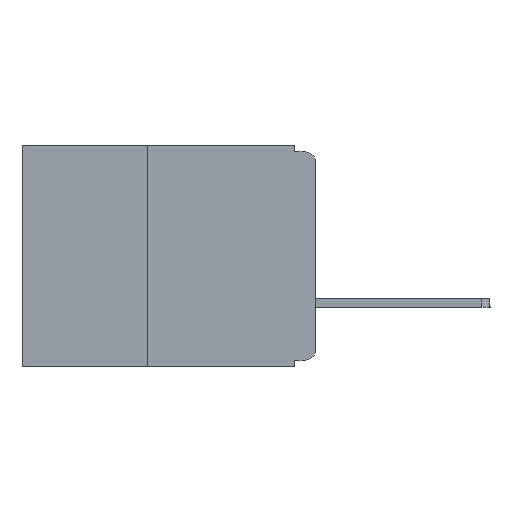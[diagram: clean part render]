
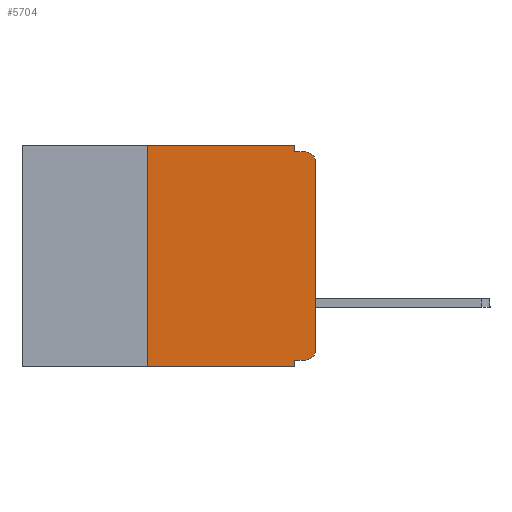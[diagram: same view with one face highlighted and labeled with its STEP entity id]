
A CAD part, left-side view. The second image highlights one B-rep face of the part: STEP entity #5704.
In plain terms, the highlighted planar face has unit normal (-1, 0, 0).
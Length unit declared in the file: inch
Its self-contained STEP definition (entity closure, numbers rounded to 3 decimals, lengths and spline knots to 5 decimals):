
#162 = EDGE_CURVE ( 'NONE', #481, #22862, #1469, .T. ) ;
#481 = VERTEX_POINT ( 'NONE', #14694 ) ;
#590 = VERTEX_POINT ( 'NONE', #20895 ) ;
#1469 = LINE ( 'NONE', #8466, #20929 ) ;
#1602 = EDGE_CURVE ( 'NONE', #24360, #5163, #13462, .T. ) ;
#1803 = ORIENTED_EDGE ( 'NONE', *, *, #17108, .F. ) ;
#2647 = EDGE_CURVE ( 'NONE', #15593, #23224, #3702, .T. ) ;
#2876 = DIRECTION ( 'NONE',  ( 0., 0., -1. ) ) ;
#3011 = DIRECTION ( 'NONE',  ( -1., 0., 0. ) ) ;
#3167 = CARTESIAN_POINT ( 'NONE',  ( 0., 0.015, -0.025 ) ) ;
#3227 = ORIENTED_EDGE ( 'NONE', *, *, #11459, .F. ) ;
#3702 = LINE ( 'NONE', #5252, #23172 ) ;
#3793 = VECTOR ( 'NONE', #11118, 39.37008 ) ;
#4370 = CARTESIAN_POINT ( 'NONE',  ( 0., 0.031, -0.33 ) ) ;
#4485 = DIRECTION ( 'NONE',  ( 1., 0., 0. ) ) ;
#5112 = DIRECTION ( 'NONE',  ( 0., 0., -1. ) ) ;
#5163 = VERTEX_POINT ( 'NONE', #10400 ) ;
#5252 = CARTESIAN_POINT ( 'NONE',  ( 0., 0., -0.32 ) ) ;
#5704 = ADVANCED_FACE ( 'NONE', ( #7215 ), #13904, .F. ) ;
#6299 = LINE ( 'NONE', #12323, #10757 ) ;
#7215 = FACE_OUTER_BOUND ( 'NONE', #22730, .T. ) ;
#7368 = CARTESIAN_POINT ( 'NONE',  ( 0., 0.031, -0.33 ) ) ;
#8285 = CARTESIAN_POINT ( 'NONE',  ( 0., 0.031, -0.01 ) ) ;
#8466 = CARTESIAN_POINT ( 'NONE',  ( 0., 0.031, 0. ) ) ;
#8816 = CARTESIAN_POINT ( 'NONE',  ( 0., 0.015, -0.305 ) ) ;
#9019 = VERTEX_POINT ( 'NONE', #7368 ) ;
#9244 = LINE ( 'NONE', #20651, #13685 ) ;
#9420 = AXIS2_PLACEMENT_3D ( 'NONE', #17643, #4485, #17721 ) ;
#9978 = EDGE_CURVE ( 'NONE', #15593, #12582, #23554, .T. ) ;
#9984 = LINE ( 'NONE', #13080, #19439 ) ;
#10085 = DIRECTION ( 'NONE',  ( 0., 0., -1. ) ) ;
#10152 = AXIS2_PLACEMENT_3D ( 'NONE', #3167, #3011, #2876 ) ;
#10177 = EDGE_CURVE ( 'NONE', #12582, #24360, #9984, .T. ) ;
#10400 = CARTESIAN_POINT ( 'NONE',  ( 0., 0.015, -0.01 ) ) ;
#10725 = DIRECTION ( 'NONE',  ( 0., 0., -1. ) ) ;
#10757 = VECTOR ( 'NONE', #23616, 39.37008 ) ;
#11118 = DIRECTION ( 'NONE',  ( 0., -1., 0. ) ) ;
#11459 = EDGE_CURVE ( 'NONE', #23224, #9019, #16341, .T. ) ;
#12323 = CARTESIAN_POINT ( 'NONE',  ( 0., 0.437, 0. ) ) ;
#12582 = VERTEX_POINT ( 'NONE', #13577 ) ;
#12796 = DIRECTION ( 'NONE',  ( 0., 1., 0. ) ) ;
#12901 = VECTOR ( 'NONE', #21005, 39.37008 ) ;
#13080 = CARTESIAN_POINT ( 'NONE',  ( 0., 0., 0. ) ) ;
#13462 = CIRCLE ( 'NONE', #10152, 0.015 ) ;
#13577 = CARTESIAN_POINT ( 'NONE',  ( 0., 0., -0.305 ) ) ;
#13685 = VECTOR ( 'NONE', #15046, 39.37008 ) ;
#13904 = PLANE ( 'NONE',  #9420 ) ;
#14694 = CARTESIAN_POINT ( 'NONE',  ( 0., 0.031, 0. ) ) ;
#15046 = DIRECTION ( 'NONE',  ( 0., 0., 1. ) ) ;
#15059 = ORIENTED_EDGE ( 'NONE', *, *, #23118, .T. ) ;
#15593 = VERTEX_POINT ( 'NONE', #18589 ) ;
#16341 = LINE ( 'NONE', #4370, #19588 ) ;
#16381 = ORIENTED_EDGE ( 'NONE', *, *, #9978, .T. ) ;
#16814 = EDGE_CURVE ( 'NONE', #590, #481, #6299, .T. ) ;
#16918 = CARTESIAN_POINT ( 'NONE',  ( 0., 0., -0.025 ) ) ;
#17108 = EDGE_CURVE ( 'NONE', #18273, #590, #9244, .T. ) ;
#17643 = CARTESIAN_POINT ( 'NONE',  ( 0., 0.437, 0. ) ) ;
#17721 = DIRECTION ( 'NONE',  ( 0., 0., -1. ) ) ;
#18273 = VERTEX_POINT ( 'NONE', #24373 ) ;
#18589 = CARTESIAN_POINT ( 'NONE',  ( 0., 0.015, -0.32 ) ) ;
#19137 = CARTESIAN_POINT ( 'NONE',  ( 0., 0., -0.01 ) ) ;
#19439 = VECTOR ( 'NONE', #22591, 39.37008 ) ;
#19588 = VECTOR ( 'NONE', #10085, 39.37008 ) ;
#20037 = AXIS2_PLACEMENT_3D ( 'NONE', #8816, #22015, #10725 ) ;
#20486 = EDGE_CURVE ( 'NONE', #22862, #5163, #22947, .T. ) ;
#20651 = CARTESIAN_POINT ( 'NONE',  ( 0., 0.25, -0.33 ) ) ;
#20895 = CARTESIAN_POINT ( 'NONE',  ( 0., 0.25, 0. ) ) ;
#20929 = VECTOR ( 'NONE', #5112, 39.37008 ) ;
#21005 = DIRECTION ( 'NONE',  ( 0., -1., 0. ) ) ;
#21114 = ORIENTED_EDGE ( 'NONE', *, *, #20486, .F. ) ;
#21127 = ORIENTED_EDGE ( 'NONE', *, *, #162, .F. ) ;
#21131 = ORIENTED_EDGE ( 'NONE', *, *, #16814, .F. ) ;
#22015 = DIRECTION ( 'NONE',  ( -1., 0., 0. ) ) ;
#22414 = CARTESIAN_POINT ( 'NONE',  ( 0., 0.437, -0.33 ) ) ;
#22500 = ORIENTED_EDGE ( 'NONE', *, *, #1602, .T. ) ;
#22507 = ORIENTED_EDGE ( 'NONE', *, *, #2647, .F. ) ;
#22591 = DIRECTION ( 'NONE',  ( 0., 0., 1. ) ) ;
#22663 = CARTESIAN_POINT ( 'NONE',  ( 0., 0.031, -0.32 ) ) ;
#22730 = EDGE_LOOP ( 'NONE', ( #23712, #22500, #21114, #21127, #21131, #1803, #15059, #3227, #22507, #16381 ) ) ;
#22862 = VERTEX_POINT ( 'NONE', #8285 ) ;
#22947 = LINE ( 'NONE', #19137, #12901 ) ;
#23118 = EDGE_CURVE ( 'NONE', #18273, #9019, #23253, .T. ) ;
#23172 = VECTOR ( 'NONE', #12796, 39.37008 ) ;
#23224 = VERTEX_POINT ( 'NONE', #22663 ) ;
#23253 = LINE ( 'NONE', #22414, #3793 ) ;
#23554 = CIRCLE ( 'NONE', #20037, 0.015 ) ;
#23616 = DIRECTION ( 'NONE',  ( 0., -1., 0. ) ) ;
#23712 = ORIENTED_EDGE ( 'NONE', *, *, #10177, .T. ) ;
#24360 = VERTEX_POINT ( 'NONE', #16918 ) ;
#24373 = CARTESIAN_POINT ( 'NONE',  ( 0., 0.25, -0.33 ) ) ;
